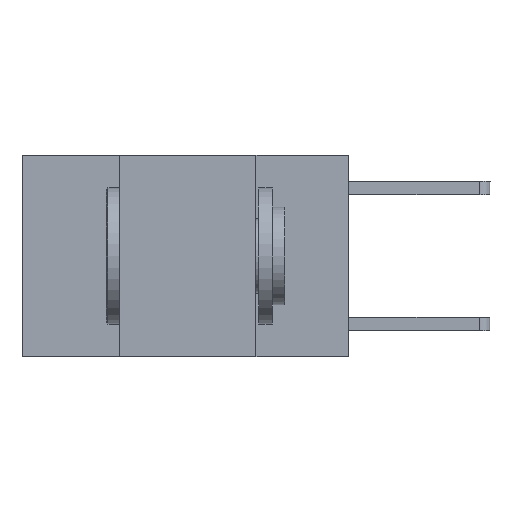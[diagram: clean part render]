
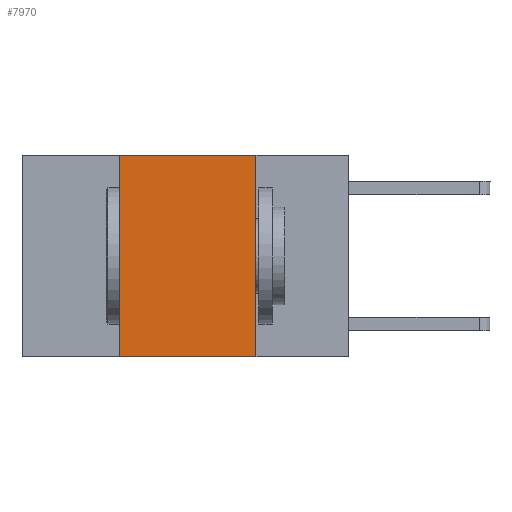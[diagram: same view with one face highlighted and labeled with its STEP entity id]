
A CAD part, left-side view. The second image highlights one B-rep face of the part: STEP entity #7970.
In plain terms, the highlighted planar face has unit normal (-1, 0, 0).
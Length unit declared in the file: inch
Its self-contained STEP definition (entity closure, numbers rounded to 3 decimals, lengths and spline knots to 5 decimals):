
#545 = VERTEX_POINT ( 'NONE', #1846 ) ;
#801 = CARTESIAN_POINT ( 'NONE',  ( 0., 0.42, 0. ) ) ;
#1008 = DIRECTION ( 'NONE',  ( 0., -1., 0. ) ) ;
#1258 = ORIENTED_EDGE ( 'NONE', *, *, #6647, .F. ) ;
#1362 = CARTESIAN_POINT ( 'NONE',  ( 0., 0.17, 0. ) ) ;
#1578 = LINE ( 'NONE', #7497, #3347 ) ;
#1579 = PLANE ( 'NONE',  #5856 ) ;
#1788 = DIRECTION ( 'NONE',  ( 0., 0., -1. ) ) ;
#1846 = CARTESIAN_POINT ( 'NONE',  ( 0., 0.17, -0.37 ) ) ;
#1998 = VERTEX_POINT ( 'NONE', #1362 ) ;
#2260 = DIRECTION ( 'NONE',  ( 0., 0., -1. ) ) ;
#2548 = LINE ( 'NONE', #6891, #5156 ) ;
#3060 = VERTEX_POINT ( 'NONE', #801 ) ;
#3347 = VECTOR ( 'NONE', #1008, 39.37008 ) ;
#3855 = VECTOR ( 'NONE', #3864, 39.37008 ) ;
#3864 = DIRECTION ( 'NONE',  ( 0., 0., 1. ) ) ;
#3923 = EDGE_CURVE ( 'NONE', #6249, #3060, #8877, .T. ) ;
#4293 = EDGE_LOOP ( 'NONE', ( #4313, #1258, #7065, #8323 ) ) ;
#4313 = ORIENTED_EDGE ( 'NONE', *, *, #7937, .F. ) ;
#4798 = VECTOR ( 'NONE', #2260, 39.37008 ) ;
#5156 = VECTOR ( 'NONE', #6990, 39.37008 ) ;
#5237 = CARTESIAN_POINT ( 'NONE',  ( 0., 0.6, 0. ) ) ;
#5334 = CARTESIAN_POINT ( 'NONE',  ( 0., 0.42, 0. ) ) ;
#5796 = EDGE_CURVE ( 'NONE', #6249, #545, #2548, .T. ) ;
#5854 = LINE ( 'NONE', #8747, #4798 ) ;
#5856 = AXIS2_PLACEMENT_3D ( 'NONE', #5237, #7405, #1788 ) ;
#6249 = VERTEX_POINT ( 'NONE', #6825 ) ;
#6647 = EDGE_CURVE ( 'NONE', #3060, #1998, #1578, .T. ) ;
#6825 = CARTESIAN_POINT ( 'NONE',  ( 0., 0.42, -0.37 ) ) ;
#6891 = CARTESIAN_POINT ( 'NONE',  ( 0., 0.6, -0.37 ) ) ;
#6990 = DIRECTION ( 'NONE',  ( 0., -1., 0. ) ) ;
#7065 = ORIENTED_EDGE ( 'NONE', *, *, #3923, .F. ) ;
#7405 = DIRECTION ( 'NONE',  ( 1., 0., 0. ) ) ;
#7497 = CARTESIAN_POINT ( 'NONE',  ( 0., 0.6, 0. ) ) ;
#7937 = EDGE_CURVE ( 'NONE', #1998, #545, #5854, .T. ) ;
#7970 = ADVANCED_FACE ( 'NONE', ( #8246 ), #1579, .F. ) ;
#8246 = FACE_OUTER_BOUND ( 'NONE', #4293, .T. ) ;
#8323 = ORIENTED_EDGE ( 'NONE', *, *, #5796, .T. ) ;
#8747 = CARTESIAN_POINT ( 'NONE',  ( 0., 0.17, 0. ) ) ;
#8877 = LINE ( 'NONE', #5334, #3855 ) ;
